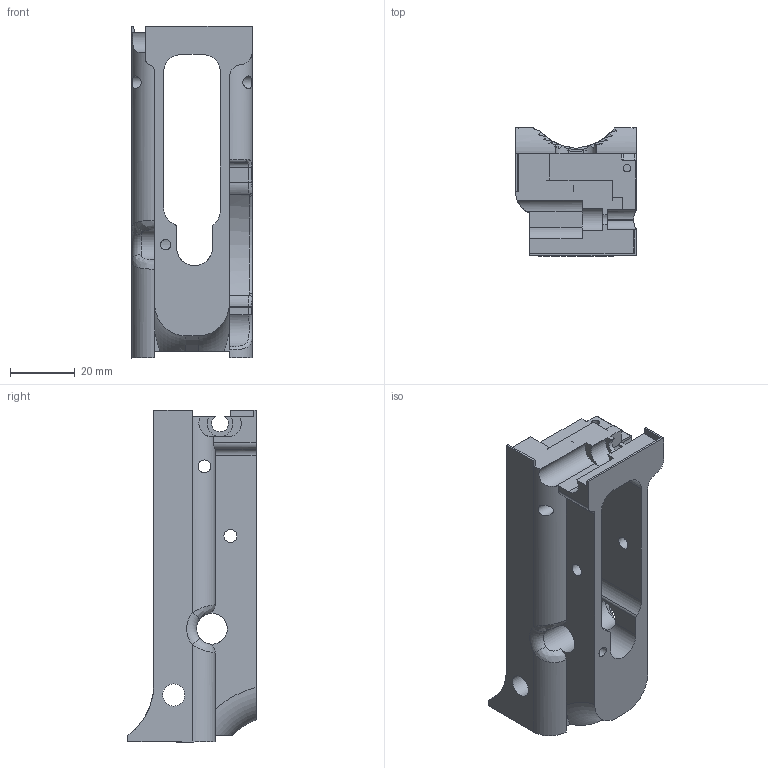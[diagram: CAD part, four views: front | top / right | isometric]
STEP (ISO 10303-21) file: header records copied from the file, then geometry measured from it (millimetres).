
FILE_DESCRIPTION (( 'STEP AP214' ), '1' );
FILE_NAME ('Hermes_v1.3.2_FCG.STEP', '2014-02-17T04:55:16', ( 'elpi' ), ( '' ), 'SwSTEP 2.0', 'SolidWorks 2013', '' );
FILE_SCHEMA (( 'AUTOMOTIVE_DESIGN' ));
Length unit declared in the file: inch
Products named in the file (1): Hermes_v1.3.2_FCG
Bounding box: 37.13 x 39.48 x 102.25 mm (x, y, z)
Volume: 52426.6 mm3; surface area: 20497 mm2
Topology: 1 solids, 1 shells, 164 faces, 472 edges, 306 vertices
Faces by surface type: cylinder 67, plane 55, bspline 30, torus 9, cone 2, sphere 1
Full cylindrical faces by diameter (mm): 2.362 x1, 3.175 x1, 3.969 x5, 6.858 x2, 9.525 x2
Entity records: 20917 total; most frequent: CARTESIAN_POINT 16904, ORIENTED_EDGE 910, DIRECTION 724, EDGE_CURVE 455, VERTEX_POINT 302, AXIS2_PLACEMENT_3D 266, EDGE_LOOP 193, LINE 192
